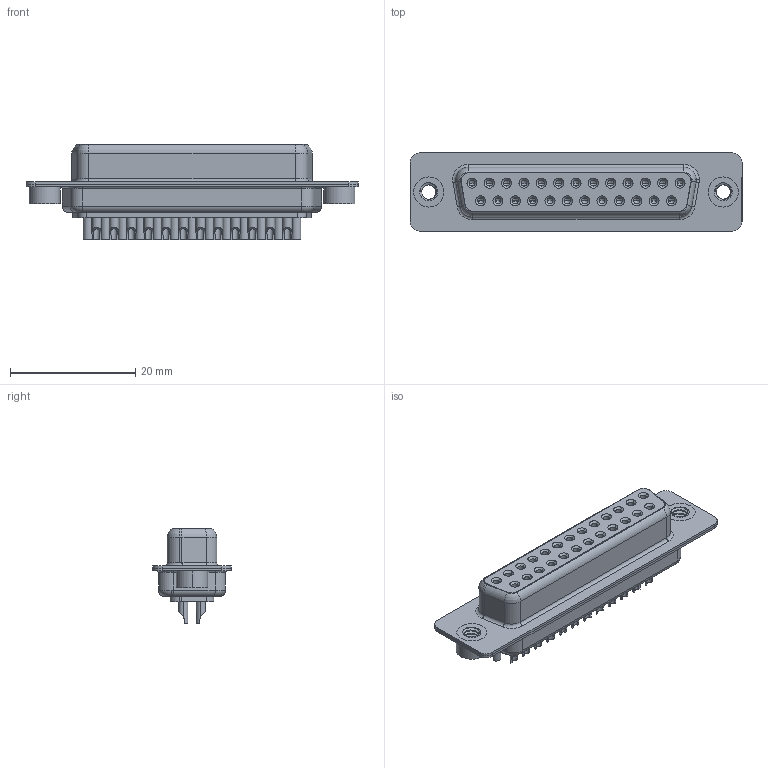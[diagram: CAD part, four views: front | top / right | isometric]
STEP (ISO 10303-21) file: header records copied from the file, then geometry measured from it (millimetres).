
FILE_DESCRIPTION (( 'STEP AP203' ), '1' );
FILE_NAME ('628-M25-222-GT2.STEP', '2021-04-26T14:04:49', ( '' ), ( '' ), 'SwSTEP 2.0', 'SolidWorks 2020', '' );
FILE_SCHEMA (( 'CONFIG_CONTROL_DESIGN' ));
Length unit declared in the file: millimetre
Products named in the file (7): 628M Shell Rear_25 Contacts; 628M Contact Row 2_22; 628M Shell Front_25 Contacts; 628-M25-222-GT2; 628M 4-40 Threaded Rivet; 628M Contact Row 1_22; 628M Housing_25 Contacts
Assembly tree (30 placements, depth 2):
  628-M25-222-GT2
    628M Housing_25 Contacts
    628M Shell Front_25 Contacts
    628M Shell Rear_25 Contacts
    628M Contact Row 1_22  x13
    628M Contact Row 2_22  x12
    628M 4-40 Threaded Rivet  x2
Bounding box: 53.05 x 12.5 x 15.25 mm (x, y, z)
Volume: 3776 mm3; surface area: 9353.6 mm2
Topology: 30 solids, 30 shells, 1655 faces, 4087 edges, 2529 vertices
Faces by surface type: cylinder 662, plane 493, torus 263, cone 231, bspline 6
Entity records: 21943 total; most frequent: CARTESIAN_POINT 4908, DIRECTION 3619, ORIENTED_EDGE 3026, AXIS2_PLACEMENT_3D 1520, EDGE_CURVE 1513, VERTEX_POINT 958, CIRCLE 834, EDGE_LOOP 809
